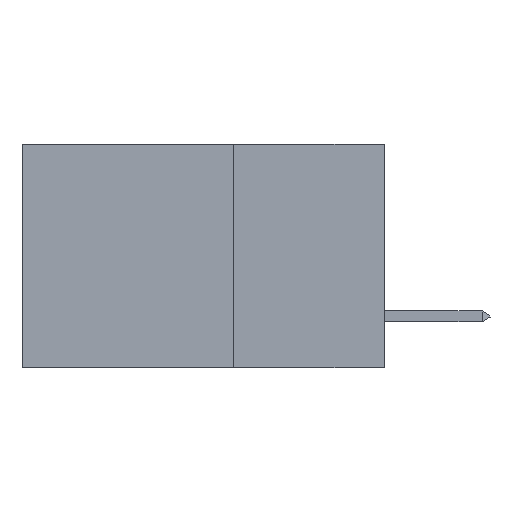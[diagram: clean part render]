
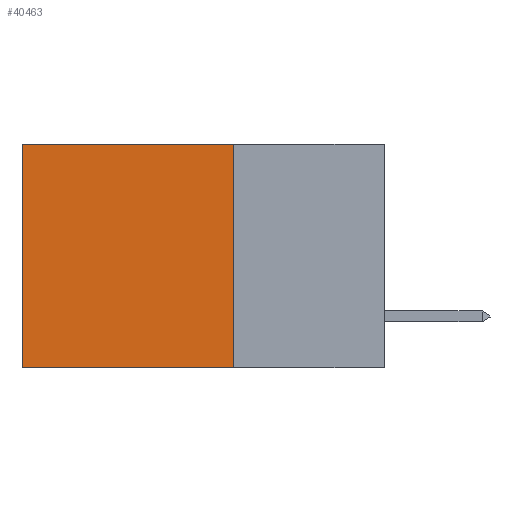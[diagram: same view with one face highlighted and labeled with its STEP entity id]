
A CAD part, left-side view. The second image highlights one B-rep face of the part: STEP entity #40463.
In plain terms, the highlighted planar face has unit normal (-1, 0, 0).
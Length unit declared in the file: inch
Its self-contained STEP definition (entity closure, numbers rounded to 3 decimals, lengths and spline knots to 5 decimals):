
#594 = ORIENTED_EDGE ( 'NONE', *, *, #35024, .T. ) ;
#1537 = LINE ( 'NONE', #19002, #2732 ) ;
#2732 = VECTOR ( 'NONE', #34261, 39.37008 ) ;
#3446 = CARTESIAN_POINT ( 'NONE',  ( 0.2875, 0.25, -0.37 ) ) ;
#5317 = ORIENTED_EDGE ( 'NONE', *, *, #31111, .F. ) ;
#5532 = FACE_OUTER_BOUND ( 'NONE', #20920, .T. ) ;
#8457 = AXIS2_PLACEMENT_3D ( 'NONE', #12309, #29333, #43701 ) ;
#10563 = ORIENTED_EDGE ( 'NONE', *, *, #14160, .F. ) ;
#11827 = ORIENTED_EDGE ( 'NONE', *, *, #24126, .T. ) ;
#12309 = CARTESIAN_POINT ( 'NONE',  ( 0.2875, 0.25, 0. ) ) ;
#14091 = VECTOR ( 'NONE', #37042, 39.37008 ) ;
#14160 = EDGE_CURVE ( 'NONE', #49237, #32530, #32939, .T. ) ;
#15755 = CARTESIAN_POINT ( 'NONE',  ( 0.2875, 0.25, 0. ) ) ;
#16598 = PLANE ( 'NONE',  #8457 ) ;
#19002 = CARTESIAN_POINT ( 'NONE',  ( 0.2875, 0.25, 0. ) ) ;
#20920 = EDGE_LOOP ( 'NONE', ( #594, #10563, #5317, #11827 ) ) ;
#21496 = VERTEX_POINT ( 'NONE', #21944 ) ;
#21944 = CARTESIAN_POINT ( 'NONE',  ( 0.2875, 0.25, 0. ) ) ;
#22373 = CARTESIAN_POINT ( 'NONE',  ( 0.2875, 0.6, 0. ) ) ;
#24126 = EDGE_CURVE ( 'NONE', #21496, #36705, #1537, .T. ) ;
#27155 = CARTESIAN_POINT ( 'NONE',  ( 0.2875, 0.6, -0.37 ) ) ;
#29333 = DIRECTION ( 'NONE',  ( 1., 0., 0. ) ) ;
#31111 = EDGE_CURVE ( 'NONE', #21496, #49237, #40657, .T. ) ;
#32530 = VERTEX_POINT ( 'NONE', #27155 ) ;
#32939 = LINE ( 'NONE', #40619, #14091 ) ;
#33556 = DIRECTION ( 'NONE',  ( 0., 0., -1. ) ) ;
#34261 = DIRECTION ( 'NONE',  ( 0., 1., 0. ) ) ;
#34760 = VECTOR ( 'NONE', #33556, 39.37008 ) ;
#35024 = EDGE_CURVE ( 'NONE', #36705, #32530, #48756, .T. ) ;
#36705 = VERTEX_POINT ( 'NONE', #22373 ) ;
#37042 = DIRECTION ( 'NONE',  ( 0., 1., 0. ) ) ;
#38232 = VECTOR ( 'NONE', #47163, 39.37008 ) ;
#40463 = ADVANCED_FACE ( 'NONE', ( #5532 ), #16598, .F. ) ;
#40619 = CARTESIAN_POINT ( 'NONE',  ( 0.2875, 0.25, -0.37 ) ) ;
#40657 = LINE ( 'NONE', #15755, #38232 ) ;
#43701 = DIRECTION ( 'NONE',  ( 0., 0., -1. ) ) ;
#45597 = CARTESIAN_POINT ( 'NONE',  ( 0.2875, 0.6, 0. ) ) ;
#47163 = DIRECTION ( 'NONE',  ( 0., 0., -1. ) ) ;
#48756 = LINE ( 'NONE', #45597, #34760 ) ;
#49237 = VERTEX_POINT ( 'NONE', #3446 ) ;
